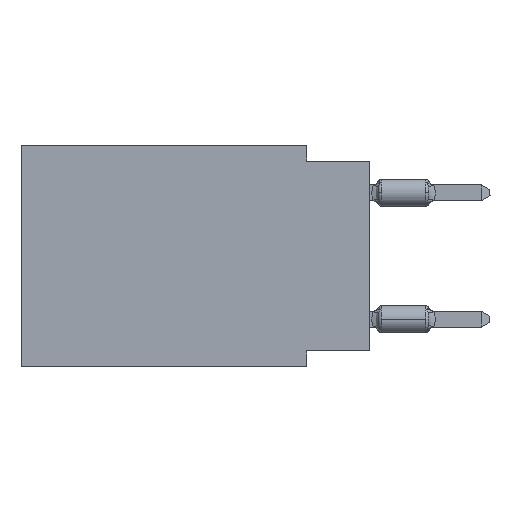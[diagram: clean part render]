
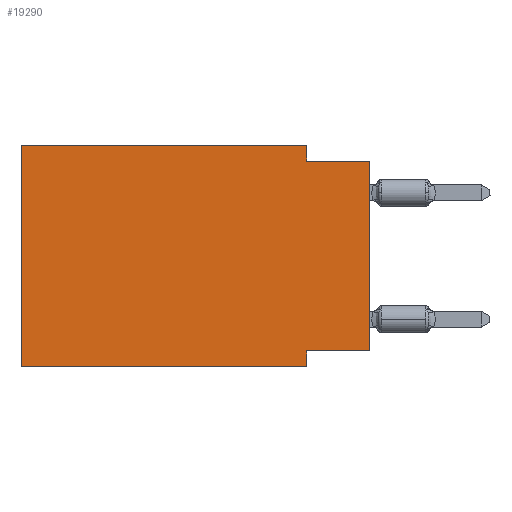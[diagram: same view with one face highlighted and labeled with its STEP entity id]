
A CAD part, left-side view. The second image highlights one B-rep face of the part: STEP entity #19290.
In plain terms, the highlighted planar face has unit normal (-1, 0, 0).
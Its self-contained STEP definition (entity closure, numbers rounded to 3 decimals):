
#361 = CARTESIAN_POINT ( 'NONE',  ( 0., 13.97, 0. ) ) ;
#823 = DIRECTION ( 'NONE',  ( 0., 1., 0. ) ) ;
#1018 = EDGE_CURVE ( 'NONE', #4163, #10715, #31198, .T. ) ;
#1531 = CARTESIAN_POINT ( 'NONE',  ( 0., 2.54, -8.89 ) ) ;
#1633 = DIRECTION ( 'NONE',  ( 0., 0., -1. ) ) ;
#1926 = CARTESIAN_POINT ( 'NONE',  ( 0., 2.54, 0. ) ) ;
#4163 = VERTEX_POINT ( 'NONE', #10769 ) ;
#6176 = VERTEX_POINT ( 'NONE', #38837 ) ;
#6793 = DIRECTION ( 'NONE',  ( 0., -1., 0. ) ) ;
#10451 = DIRECTION ( 'NONE',  ( 0., -1., 0. ) ) ;
#10715 = VERTEX_POINT ( 'NONE', #29216 ) ;
#10761 = VECTOR ( 'NONE', #823, 1000. ) ;
#10769 = CARTESIAN_POINT ( 'NONE',  ( 0., 2.54, -8.255 ) ) ;
#11810 = ORIENTED_EDGE ( 'NONE', *, *, #29649, .T. ) ;
#13827 = EDGE_CURVE ( 'NONE', #29724, #37859, #61654, .T. ) ;
#14936 = CARTESIAN_POINT ( 'NONE',  ( 0., 13.97, -8.89 ) ) ;
#15201 = VECTOR ( 'NONE', #1633, 1000. ) ;
#15605 = ORIENTED_EDGE ( 'NONE', *, *, #19107, .F. ) ;
#16385 = ORIENTED_EDGE ( 'NONE', *, *, #13827, .F. ) ;
#16882 = LINE ( 'NONE', #61304, #31989 ) ;
#16924 = CARTESIAN_POINT ( 'NONE',  ( 0., 2.54, 0. ) ) ;
#18016 = AXIS2_PLACEMENT_3D ( 'NONE', #36980, #41242, #37313 ) ;
#18733 = CARTESIAN_POINT ( 'NONE',  ( 0., 0., -0.635 ) ) ;
#19084 = EDGE_LOOP ( 'NONE', ( #31545, #52209, #16385, #51246, #32726, #11810, #44029, #15605 ) ) ;
#19107 = EDGE_CURVE ( 'NONE', #36152, #4163, #55296, .T. ) ;
#19269 = VECTOR ( 'NONE', #10451, 1000. ) ;
#19290 = ADVANCED_FACE ( 'NONE', ( #31443 ), #32411, .F. ) ;
#20216 = LINE ( 'NONE', #49927, #21160 ) ;
#21160 = VECTOR ( 'NONE', #45336, 1000. ) ;
#23622 = DIRECTION ( 'NONE',  ( 0., -1., 0. ) ) ;
#25648 = DIRECTION ( 'NONE',  ( 0., 0., -1. ) ) ;
#27513 = CARTESIAN_POINT ( 'NONE',  ( 0., 13.97, 0. ) ) ;
#29216 = CARTESIAN_POINT ( 'NONE',  ( 0., 2.54, -8.89 ) ) ;
#29649 = EDGE_CURVE ( 'NONE', #35966, #10715, #16882, .T. ) ;
#29724 = VERTEX_POINT ( 'NONE', #1926 ) ;
#31198 = LINE ( 'NONE', #1531, #50800 ) ;
#31443 = FACE_OUTER_BOUND ( 'NONE', #19084, .T. ) ;
#31545 = ORIENTED_EDGE ( 'NONE', *, *, #46496, .T. ) ;
#31989 = VECTOR ( 'NONE', #6793, 1000. ) ;
#32408 = LINE ( 'NONE', #27513, #54177 ) ;
#32411 = PLANE ( 'NONE',  #18016 ) ;
#32726 = ORIENTED_EDGE ( 'NONE', *, *, #47612, .F. ) ;
#35966 = VERTEX_POINT ( 'NONE', #14936 ) ;
#36012 = CARTESIAN_POINT ( 'NONE',  ( 0., 0., -8.255 ) ) ;
#36152 = VERTEX_POINT ( 'NONE', #38698 ) ;
#36643 = EDGE_CURVE ( 'NONE', #37859, #44049, #48417, .T. ) ;
#36980 = CARTESIAN_POINT ( 'NONE',  ( 0., 13.97, 0. ) ) ;
#37313 = DIRECTION ( 'NONE',  ( 0., 0., -1. ) ) ;
#37859 = VERTEX_POINT ( 'NONE', #53255 ) ;
#38698 = CARTESIAN_POINT ( 'NONE',  ( 0., 0., -8.255 ) ) ;
#38837 = CARTESIAN_POINT ( 'NONE',  ( 0., 13.97, 0. ) ) ;
#41242 = DIRECTION ( 'NONE',  ( 1., 0., 0. ) ) ;
#44029 = ORIENTED_EDGE ( 'NONE', *, *, #1018, .F. ) ;
#44049 = VERTEX_POINT ( 'NONE', #18733 ) ;
#45336 = DIRECTION ( 'NONE',  ( 0., 0., 1. ) ) ;
#46496 = EDGE_CURVE ( 'NONE', #36152, #44049, #20216, .T. ) ;
#47612 = EDGE_CURVE ( 'NONE', #35966, #6176, #32408, .T. ) ;
#48417 = LINE ( 'NONE', #53315, #48431 ) ;
#48431 = VECTOR ( 'NONE', #23622, 1000. ) ;
#49927 = CARTESIAN_POINT ( 'NONE',  ( 0., 0., 0. ) ) ;
#50800 = VECTOR ( 'NONE', #25648, 1000. ) ;
#51246 = ORIENTED_EDGE ( 'NONE', *, *, #61679, .F. ) ;
#52209 = ORIENTED_EDGE ( 'NONE', *, *, #36643, .F. ) ;
#53255 = CARTESIAN_POINT ( 'NONE',  ( 0., 2.54, -0.635 ) ) ;
#53315 = CARTESIAN_POINT ( 'NONE',  ( 0., 0., -0.635 ) ) ;
#54177 = VECTOR ( 'NONE', #57547, 1000. ) ;
#55296 = LINE ( 'NONE', #36012, #10761 ) ;
#55472 = LINE ( 'NONE', #361, #19269 ) ;
#57547 = DIRECTION ( 'NONE',  ( 0., 0., 1. ) ) ;
#61304 = CARTESIAN_POINT ( 'NONE',  ( 0., 13.97, -8.89 ) ) ;
#61654 = LINE ( 'NONE', #16924, #15201 ) ;
#61679 = EDGE_CURVE ( 'NONE', #6176, #29724, #55472, .T. ) ;
